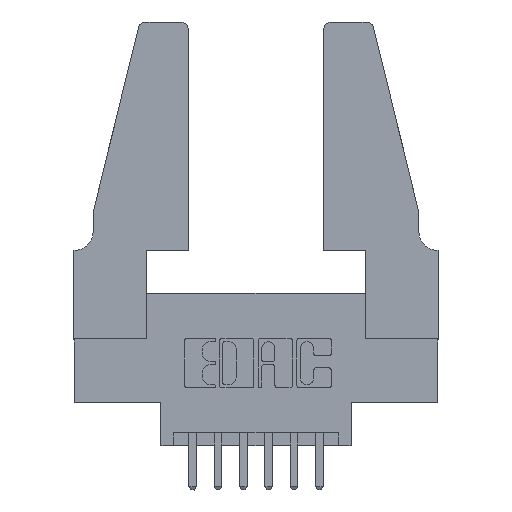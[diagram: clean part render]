
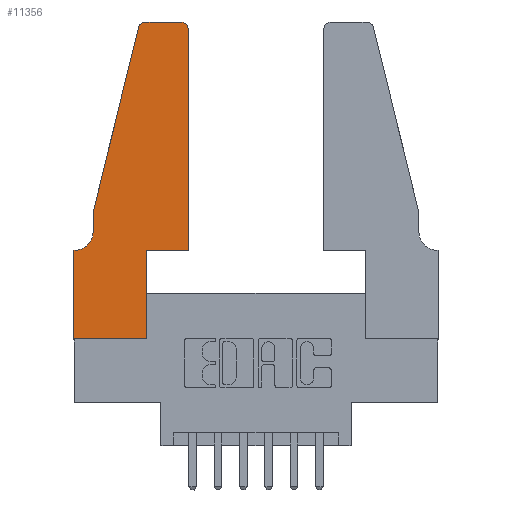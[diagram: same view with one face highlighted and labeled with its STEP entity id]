
A CAD part, top view. The second image highlights one B-rep face of the part: STEP entity #11356.
In plain terms, the highlighted planar face has unit normal (0, 0, 1).
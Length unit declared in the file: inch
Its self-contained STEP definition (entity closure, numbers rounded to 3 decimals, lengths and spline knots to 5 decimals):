
#75 = EDGE_CURVE ( 'NONE', #9471, #786, #11074, .T. ) ;
#142 = LINE ( 'NONE', #1991, #1127 ) ;
#301 = EDGE_CURVE ( 'NONE', #786, #485, #5585, .T. ) ;
#312 = DIRECTION ( 'NONE',  ( 0., -1., 0. ) ) ;
#448 = ORIENTED_EDGE ( 'NONE', *, *, #10101, .T. ) ;
#485 = VERTEX_POINT ( 'NONE', #8389 ) ;
#615 = PLANE ( 'NONE',  #4539 ) ;
#670 = EDGE_CURVE ( 'NONE', #3709, #4001, #5735, .T. ) ;
#786 = VERTEX_POINT ( 'NONE', #3680 ) ;
#806 = LINE ( 'NONE', #6082, #1634 ) ;
#834 = VERTEX_POINT ( 'NONE', #1814 ) ;
#939 = DIRECTION ( 'NONE',  ( 1., 0., 0. ) ) ;
#946 = LINE ( 'NONE', #6206, #10483 ) ;
#1031 = DIRECTION ( 'NONE',  ( 0., 1., 0. ) ) ;
#1127 = VECTOR ( 'NONE', #1146, 39.37008 ) ;
#1146 = DIRECTION ( 'NONE',  ( 0., -1., 0. ) ) ;
#1243 = VECTOR ( 'NONE', #4316, 39.37008 ) ;
#1611 = VECTOR ( 'NONE', #939, 39.37008 ) ;
#1634 = VECTOR ( 'NONE', #2189, 39.37008 ) ;
#1783 = ORIENTED_EDGE ( 'NONE', *, *, #10804, .T. ) ;
#1814 = CARTESIAN_POINT ( 'NONE',  ( 0., 0., 0.37 ) ) ;
#1991 = CARTESIAN_POINT ( 'NONE',  ( 0., 0., 0.37 ) ) ;
#2062 = ORIENTED_EDGE ( 'NONE', *, *, #75, .T. ) ;
#2145 = VERTEX_POINT ( 'NONE', #5390 ) ;
#2189 = DIRECTION ( 'NONE',  ( -0.239, -0.971, 0. ) ) ;
#2204 = CARTESIAN_POINT ( 'NONE',  ( 0.0055, 0.42, 0.37 ) ) ;
#2529 = DIRECTION ( 'NONE',  ( -1., 0., 0. ) ) ;
#2774 = ORIENTED_EDGE ( 'NONE', *, *, #5605, .T. ) ;
#2967 = DIRECTION ( 'NONE',  ( -1., 0., 0. ) ) ;
#3219 = CARTESIAN_POINT ( 'NONE',  ( 0.2865, 0.35, 0.37 ) ) ;
#3347 = VERTEX_POINT ( 'NONE', #6887 ) ;
#3377 = AXIS2_PLACEMENT_3D ( 'NONE', #2204, #4085, #11497 ) ;
#3390 = DIRECTION ( 'NONE',  ( 1., 0., 0. ) ) ;
#3436 = EDGE_CURVE ( 'NONE', #3347, #5803, #4637, .T. ) ;
#3658 = CARTESIAN_POINT ( 'NONE',  ( 0.4505, 0.35, 0.37 ) ) ;
#3680 = CARTESIAN_POINT ( 'NONE',  ( 0.4505, 1.22, 0.37 ) ) ;
#3709 = VERTEX_POINT ( 'NONE', #8445 ) ;
#3790 = CARTESIAN_POINT ( 'NONE',  ( 0., 0., 0.37 ) ) ;
#4001 = VERTEX_POINT ( 'NONE', #3219 ) ;
#4085 = DIRECTION ( 'NONE',  ( 0., 0., -1. ) ) ;
#4284 = EDGE_CURVE ( 'NONE', #485, #8436, #8982, .T. ) ;
#4316 = DIRECTION ( 'NONE',  ( 0., 1., 0. ) ) ;
#4426 = AXIS2_PLACEMENT_3D ( 'NONE', #7193, #8030, #3390 ) ;
#4539 = AXIS2_PLACEMENT_3D ( 'NONE', #8819, #9861, #6195 ) ;
#4637 = CIRCLE ( 'NONE', #3377, 0.07 ) ;
#4888 = CIRCLE ( 'NONE', #4426, 0.03 ) ;
#4979 = ORIENTED_EDGE ( 'NONE', *, *, #670, .T. ) ;
#5053 = VECTOR ( 'NONE', #2529, 39.37008 ) ;
#5214 = CARTESIAN_POINT ( 'NONE',  ( 0.2865, 0.35, 0.37 ) ) ;
#5216 = CARTESIAN_POINT ( 'NONE',  ( 0.2605, 1.25, 0.37 ) ) ;
#5363 = ORIENTED_EDGE ( 'NONE', *, *, #6097, .T. ) ;
#5369 = DIRECTION ( 'NONE',  ( 1., 0., 0. ) ) ;
#5390 = CARTESIAN_POINT ( 'NONE',  ( 0.0755, 0.5, 0.37 ) ) ;
#5585 = CIRCLE ( 'NONE', #6788, 0.03 ) ;
#5605 = EDGE_CURVE ( 'NONE', #7529, #834, #142, .T. ) ;
#5672 = LINE ( 'NONE', #3790, #1611 ) ;
#5693 = FACE_OUTER_BOUND ( 'NONE', #5873, .T. ) ;
#5735 = LINE ( 'NONE', #5214, #1243 ) ;
#5803 = VERTEX_POINT ( 'NONE', #8783 ) ;
#5829 = CARTESIAN_POINT ( 'NONE',  ( 0.0755, 0.5, 0.37 ) ) ;
#5873 = EDGE_LOOP ( 'NONE', ( #7580, #8107, #1783, #9898, #8408, #7230, #2774, #5363, #4979, #448, #2062, #7818 ) ) ;
#6082 = CARTESIAN_POINT ( 'NONE',  ( 0.0755, 0.5, 0.37 ) ) ;
#6097 = EDGE_CURVE ( 'NONE', #834, #3709, #5672, .T. ) ;
#6195 = DIRECTION ( 'NONE',  ( 1., 0., 0. ) ) ;
#6206 = CARTESIAN_POINT ( 'NONE',  ( 0.4505, 0.35, 0.37 ) ) ;
#6788 = AXIS2_PLACEMENT_3D ( 'NONE', #11726, #9051, #5369 ) ;
#6887 = CARTESIAN_POINT ( 'NONE',  ( 0.0755, 0.42, 0.37 ) ) ;
#7193 = CARTESIAN_POINT ( 'NONE',  ( 0.284, 1.22, 0.37 ) ) ;
#7230 = ORIENTED_EDGE ( 'NONE', *, *, #11166, .T. ) ;
#7529 = VERTEX_POINT ( 'NONE', #10996 ) ;
#7580 = ORIENTED_EDGE ( 'NONE', *, *, #4284, .T. ) ;
#7818 = ORIENTED_EDGE ( 'NONE', *, *, #301, .T. ) ;
#7865 = EDGE_CURVE ( 'NONE', #2145, #3347, #10115, .T. ) ;
#7961 = EDGE_CURVE ( 'NONE', #8436, #8663, #4888, .T. ) ;
#8030 = DIRECTION ( 'NONE',  ( 0., 0., 1. ) ) ;
#8107 = ORIENTED_EDGE ( 'NONE', *, *, #7961, .T. ) ;
#8389 = CARTESIAN_POINT ( 'NONE',  ( 0.4205, 1.25, 0.37 ) ) ;
#8408 = ORIENTED_EDGE ( 'NONE', *, *, #3436, .T. ) ;
#8436 = VERTEX_POINT ( 'NONE', #10955 ) ;
#8445 = CARTESIAN_POINT ( 'NONE',  ( 0.2865, 0., 0.37 ) ) ;
#8466 = CARTESIAN_POINT ( 'NONE',  ( 0.0755, 0.35, 0.37 ) ) ;
#8622 = VECTOR ( 'NONE', #2967, 39.37008 ) ;
#8663 = VERTEX_POINT ( 'NONE', #11068 ) ;
#8678 = CARTESIAN_POINT ( 'NONE',  ( 0.4505, 0.35, 0.37 ) ) ;
#8775 = VECTOR ( 'NONE', #1031, 39.37008 ) ;
#8783 = CARTESIAN_POINT ( 'NONE',  ( 0.0055, 0.35, 0.37 ) ) ;
#8819 = CARTESIAN_POINT ( 'NONE',  ( 0., 0.35, 0.37 ) ) ;
#8952 = DIRECTION ( 'NONE',  ( 1., 0., 0. ) ) ;
#8982 = LINE ( 'NONE', #5216, #5053 ) ;
#9051 = DIRECTION ( 'NONE',  ( 0., 0., 1. ) ) ;
#9471 = VERTEX_POINT ( 'NONE', #8678 ) ;
#9861 = DIRECTION ( 'NONE',  ( 0., 0., 1. ) ) ;
#9898 = ORIENTED_EDGE ( 'NONE', *, *, #7865, .T. ) ;
#10101 = EDGE_CURVE ( 'NONE', #4001, #9471, #946, .T. ) ;
#10115 = LINE ( 'NONE', #5829, #11115 ) ;
#10483 = VECTOR ( 'NONE', #8952, 39.37008 ) ;
#10804 = EDGE_CURVE ( 'NONE', #8663, #2145, #806, .T. ) ;
#10955 = CARTESIAN_POINT ( 'NONE',  ( 0.284, 1.25, 0.37 ) ) ;
#10996 = CARTESIAN_POINT ( 'NONE',  ( 0., 0.35, 0.37 ) ) ;
#11068 = CARTESIAN_POINT ( 'NONE',  ( 0.25487, 1.22718, 0.37 ) ) ;
#11074 = LINE ( 'NONE', #3658, #8775 ) ;
#11115 = VECTOR ( 'NONE', #312, 39.37008 ) ;
#11166 = EDGE_CURVE ( 'NONE', #5803, #7529, #11339, .T. ) ;
#11339 = LINE ( 'NONE', #8466, #8622 ) ;
#11356 = ADVANCED_FACE ( 'NONE', ( #5693 ), #615, .T. ) ;
#11497 = DIRECTION ( 'NONE',  ( -1., 0., 0. ) ) ;
#11726 = CARTESIAN_POINT ( 'NONE',  ( 0.4205, 1.22, 0.37 ) ) ;
